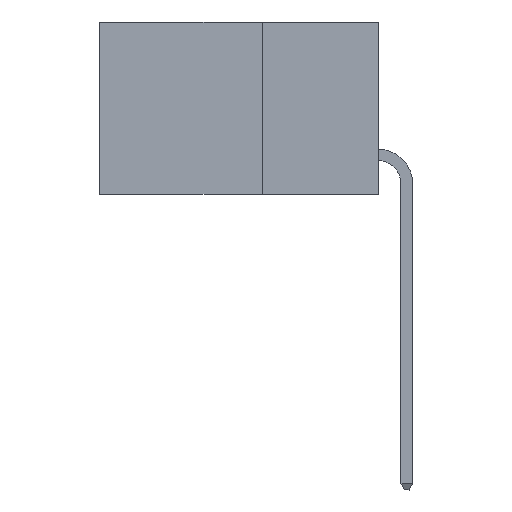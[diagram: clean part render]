
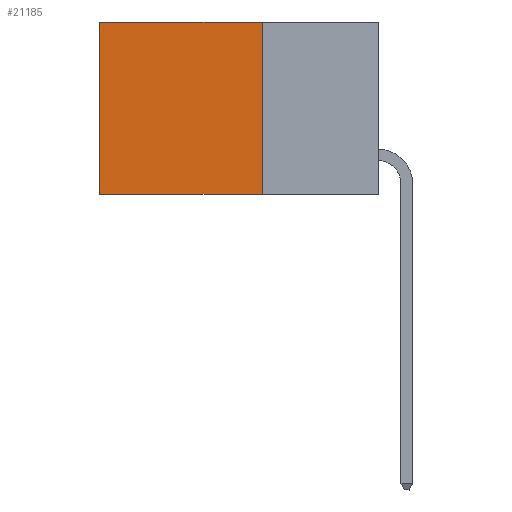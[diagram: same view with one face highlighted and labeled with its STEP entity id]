
A CAD part, left-side view. The second image highlights one B-rep face of the part: STEP entity #21185.
In plain terms, the highlighted planar face has unit normal (-1, 0, 0).
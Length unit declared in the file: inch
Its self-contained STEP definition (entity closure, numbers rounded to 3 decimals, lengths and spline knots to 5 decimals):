
#1128 = VERTEX_POINT ( 'NONE', #18499 ) ;
#1503 = CARTESIAN_POINT ( 'NONE',  ( 0.298, 0.6, 0. ) ) ;
#1873 = LINE ( 'NONE', #22408, #11820 ) ;
#2200 = EDGE_CURVE ( 'NONE', #1128, #9542, #24613, .T. ) ;
#2225 = CARTESIAN_POINT ( 'NONE',  ( 0.298, 0.25, -0.37 ) ) ;
#4148 = VECTOR ( 'NONE', #13293, 39.37008 ) ;
#4791 = LINE ( 'NONE', #18994, #4148 ) ;
#7096 = EDGE_CURVE ( 'NONE', #9542, #11122, #4791, .T. ) ;
#7402 = ORIENTED_EDGE ( 'NONE', *, *, #2200, .F. ) ;
#7691 = CARTESIAN_POINT ( 'NONE',  ( 0.298, 0.25, 0. ) ) ;
#7732 = EDGE_LOOP ( 'NONE', ( #12239, #23950, #7402, #15703 ) ) ;
#8530 = VERTEX_POINT ( 'NONE', #9527 ) ;
#9239 = DIRECTION ( 'NONE',  ( 0., 0., -1. ) ) ;
#9273 = VECTOR ( 'NONE', #9239, 39.37008 ) ;
#9398 = DIRECTION ( 'NONE',  ( 0., 0., -1. ) ) ;
#9527 = CARTESIAN_POINT ( 'NONE',  ( 0.298, 0.6, 0. ) ) ;
#9542 = VERTEX_POINT ( 'NONE', #2225 ) ;
#9551 = LINE ( 'NONE', #1503, #13548 ) ;
#9995 = AXIS2_PLACEMENT_3D ( 'NONE', #24838, #11551, #24917 ) ;
#10953 = CARTESIAN_POINT ( 'NONE',  ( 0.298, 0.6, -0.37 ) ) ;
#11122 = VERTEX_POINT ( 'NONE', #10953 ) ;
#11551 = DIRECTION ( 'NONE',  ( 1., 0., 0. ) ) ;
#11820 = VECTOR ( 'NONE', #14836, 39.37008 ) ;
#12239 = ORIENTED_EDGE ( 'NONE', *, *, #20586, .T. ) ;
#12290 = FACE_OUTER_BOUND ( 'NONE', #7732, .T. ) ;
#13293 = DIRECTION ( 'NONE',  ( 0., 1., 0. ) ) ;
#13548 = VECTOR ( 'NONE', #9398, 39.37008 ) ;
#14836 = DIRECTION ( 'NONE',  ( 0., 1., 0. ) ) ;
#15703 = ORIENTED_EDGE ( 'NONE', *, *, #19015, .T. ) ;
#18499 = CARTESIAN_POINT ( 'NONE',  ( 0.298, 0.25, 0. ) ) ;
#18994 = CARTESIAN_POINT ( 'NONE',  ( 0.298, 0.25, -0.37 ) ) ;
#19015 = EDGE_CURVE ( 'NONE', #1128, #8530, #1873, .T. ) ;
#20586 = EDGE_CURVE ( 'NONE', #8530, #11122, #9551, .T. ) ;
#21185 = ADVANCED_FACE ( 'NONE', ( #12290 ), #23010, .F. ) ;
#22408 = CARTESIAN_POINT ( 'NONE',  ( 0.298, 0.25, 0. ) ) ;
#23010 = PLANE ( 'NONE',  #9995 ) ;
#23950 = ORIENTED_EDGE ( 'NONE', *, *, #7096, .F. ) ;
#24613 = LINE ( 'NONE', #7691, #9273 ) ;
#24838 = CARTESIAN_POINT ( 'NONE',  ( 0.298, 0.25, 0. ) ) ;
#24917 = DIRECTION ( 'NONE',  ( 0., 0., -1. ) ) ;
